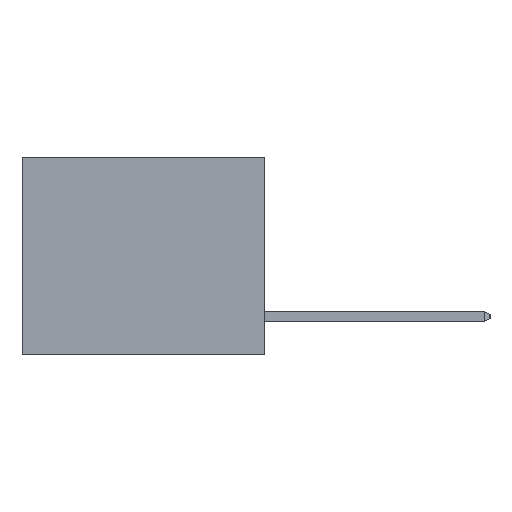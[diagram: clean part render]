
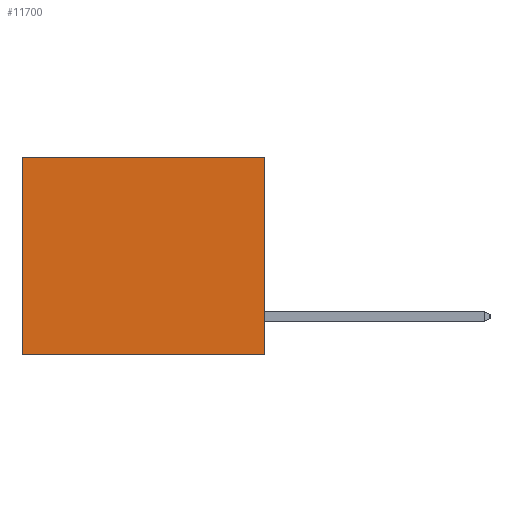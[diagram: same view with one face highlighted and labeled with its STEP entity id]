
A CAD part, left-side view. The second image highlights one B-rep face of the part: STEP entity #11700.
In plain terms, the highlighted planar face has unit normal (-1, 0, 0).
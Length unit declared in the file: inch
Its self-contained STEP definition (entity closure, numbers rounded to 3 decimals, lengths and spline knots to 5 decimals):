
#1095 = DIRECTION ( 'NONE',  ( 0., 0., -1. ) ) ;
#1187 = VECTOR ( 'NONE', #11939, 39.37008 ) ;
#3279 = EDGE_CURVE ( 'NONE', #13879, #7543, #4165, .T. ) ;
#3384 = CARTESIAN_POINT ( 'NONE',  ( 0.3165, 0., 0. ) ) ;
#3996 = AXIS2_PLACEMENT_3D ( 'NONE', #11201, #14296, #1095 ) ;
#4048 = PLANE ( 'NONE',  #3996 ) ;
#4158 = CARTESIAN_POINT ( 'NONE',  ( 0.3165, 0., -0.49 ) ) ;
#4165 = LINE ( 'NONE', #13248, #15008 ) ;
#4405 = LINE ( 'NONE', #10339, #1187 ) ;
#4974 = ORIENTED_EDGE ( 'NONE', *, *, #3279, .F. ) ;
#5202 = CARTESIAN_POINT ( 'NONE',  ( 0.3165, 0., 0. ) ) ;
#5955 = CARTESIAN_POINT ( 'NONE',  ( 0.3165, 0.6, 0. ) ) ;
#6000 = VECTOR ( 'NONE', #17055, 39.37008 ) ;
#6936 = CARTESIAN_POINT ( 'NONE',  ( 0.3165, 0., -0.49 ) ) ;
#7543 = VERTEX_POINT ( 'NONE', #6936 ) ;
#8749 = VERTEX_POINT ( 'NONE', #10266 ) ;
#9124 = EDGE_LOOP ( 'NONE', ( #12474, #19013, #4974, #18151 ) ) ;
#9243 = EDGE_CURVE ( 'NONE', #7543, #8749, #17671, .T. ) ;
#9951 = LINE ( 'NONE', #5202, #6000 ) ;
#10266 = CARTESIAN_POINT ( 'NONE',  ( 0.3165, 0.6, -0.49 ) ) ;
#10339 = CARTESIAN_POINT ( 'NONE',  ( 0.3165, 0.6, -0.49 ) ) ;
#10541 = EDGE_CURVE ( 'NONE', #13879, #12213, #9951, .T. ) ;
#11201 = CARTESIAN_POINT ( 'NONE',  ( 0.3165, 0., -0.49 ) ) ;
#11700 = ADVANCED_FACE ( 'NONE', ( #13148 ), #4048, .F. ) ;
#11939 = DIRECTION ( 'NONE',  ( 0., 0., -1. ) ) ;
#12213 = VERTEX_POINT ( 'NONE', #5955 ) ;
#12474 = ORIENTED_EDGE ( 'NONE', *, *, #14302, .T. ) ;
#13148 = FACE_OUTER_BOUND ( 'NONE', #9124, .T. ) ;
#13248 = CARTESIAN_POINT ( 'NONE',  ( 0.3165, 0., -0.49 ) ) ;
#13879 = VERTEX_POINT ( 'NONE', #3384 ) ;
#14296 = DIRECTION ( 'NONE',  ( 1., 0., 0. ) ) ;
#14302 = EDGE_CURVE ( 'NONE', #12213, #8749, #4405, .T. ) ;
#14505 = DIRECTION ( 'NONE',  ( 0., 1., 0. ) ) ;
#14723 = DIRECTION ( 'NONE',  ( 0., 0., -1. ) ) ;
#15008 = VECTOR ( 'NONE', #14723, 39.37008 ) ;
#17055 = DIRECTION ( 'NONE',  ( 0., 1., 0. ) ) ;
#17671 = LINE ( 'NONE', #4158, #18841 ) ;
#18151 = ORIENTED_EDGE ( 'NONE', *, *, #10541, .T. ) ;
#18841 = VECTOR ( 'NONE', #14505, 39.37008 ) ;
#19013 = ORIENTED_EDGE ( 'NONE', *, *, #9243, .F. ) ;
